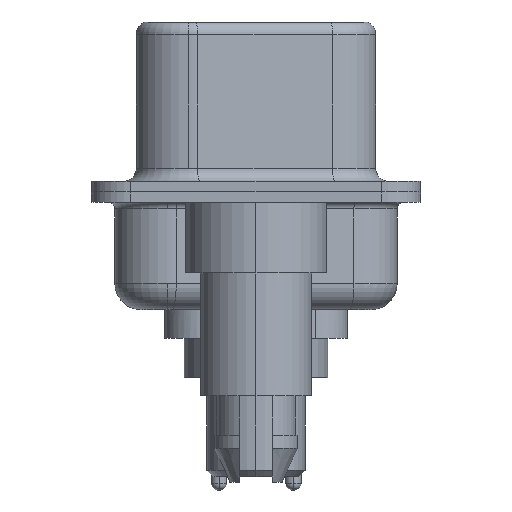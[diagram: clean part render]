
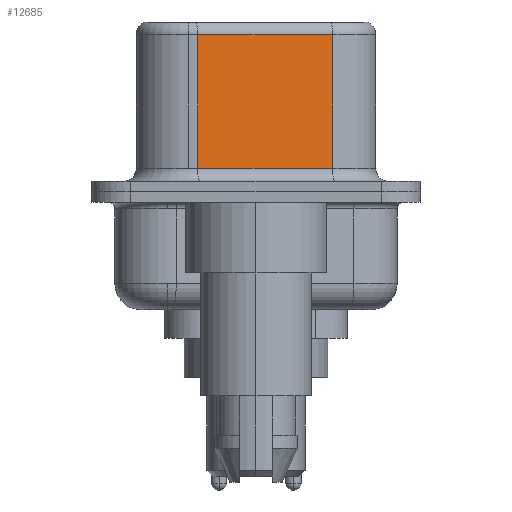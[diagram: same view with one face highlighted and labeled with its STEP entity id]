
A CAD part, left-side view. The second image highlights one B-rep face of the part: STEP entity #12685.
In plain terms, the highlighted planar face has unit normal (-0.985, -0.174, 0).
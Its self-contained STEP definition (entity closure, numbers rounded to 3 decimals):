
#523 = DIRECTION ( 'NONE',  ( -0.174, 0.985, 0. ) ) ;
#1346 = CARTESIAN_POINT ( 'NONE',  ( 4.565, -2.927, 0.9 ) ) ;
#1557 = VECTOR ( 'NONE', #4363, 1000. ) ;
#1841 = VERTEX_POINT ( 'NONE', #9374 ) ;
#3157 = LINE ( 'NONE', #1346, #6806 ) ;
#3187 = EDGE_LOOP ( 'NONE', ( #12131, #6915, #15835, #7093 ) ) ;
#3683 = CARTESIAN_POINT ( 'NONE',  ( 4.565, -2.927, 0.9 ) ) ;
#3918 = CARTESIAN_POINT ( 'NONE',  ( 4.565, -2.927, 6.02 ) ) ;
#4363 = DIRECTION ( 'NONE',  ( -0.174, 0.985, 0. ) ) ;
#4474 = VERTEX_POINT ( 'NONE', #3683 ) ;
#4487 = DIRECTION ( 'NONE',  ( 0.174, -0.985, 0. ) ) ;
#4909 = CARTESIAN_POINT ( 'NONE',  ( 3.655, 2.233, 0.9 ) ) ;
#5028 = EDGE_CURVE ( 'NONE', #8208, #1841, #9851, .T. ) ;
#5244 = EDGE_CURVE ( 'NONE', #8208, #4474, #16447, .T. ) ;
#6169 = LINE ( 'NONE', #18229, #14682 ) ;
#6806 = VECTOR ( 'NONE', #4487, 1000. ) ;
#6915 = ORIENTED_EDGE ( 'NONE', *, *, #5028, .T. ) ;
#6930 = EDGE_CURVE ( 'NONE', #1841, #20203, #6169, .T. ) ;
#7018 = DIRECTION ( 'NONE',  ( 0., 0., -1. ) ) ;
#7093 = ORIENTED_EDGE ( 'NONE', *, *, #18144, .T. ) ;
#8208 = VERTEX_POINT ( 'NONE', #3918 ) ;
#8333 = PLANE ( 'NONE',  #10334 ) ;
#9374 = CARTESIAN_POINT ( 'NONE',  ( 3.655, 2.233, 6.02 ) ) ;
#9851 = LINE ( 'NONE', #15745, #1557 ) ;
#9900 = DIRECTION ( 'NONE',  ( 0.985, 0.174, 0. ) ) ;
#10108 = DIRECTION ( 'NONE',  ( 0., 0., -1. ) ) ;
#10334 = AXIS2_PLACEMENT_3D ( 'NONE', #19604, #9900, #523 ) ;
#11743 = FACE_OUTER_BOUND ( 'NONE', #3187, .T. ) ;
#12131 = ORIENTED_EDGE ( 'NONE', *, *, #5244, .F. ) ;
#12685 = ADVANCED_FACE ( 'NONE', ( #11743 ), #8333, .F. ) ;
#14682 = VECTOR ( 'NONE', #10108, 1000. ) ;
#15432 = VECTOR ( 'NONE', #7018, 1000. ) ;
#15456 = CARTESIAN_POINT ( 'NONE',  ( 4.565, -2.927, 6.52 ) ) ;
#15745 = CARTESIAN_POINT ( 'NONE',  ( 4.565, -2.927, 6.02 ) ) ;
#15835 = ORIENTED_EDGE ( 'NONE', *, *, #6930, .T. ) ;
#16447 = LINE ( 'NONE', #15456, #15432 ) ;
#18144 = EDGE_CURVE ( 'NONE', #20203, #4474, #3157, .T. ) ;
#18229 = CARTESIAN_POINT ( 'NONE',  ( 3.655, 2.233, 6.52 ) ) ;
#19604 = CARTESIAN_POINT ( 'NONE',  ( 4.565, -2.927, 6.52 ) ) ;
#20203 = VERTEX_POINT ( 'NONE', #4909 ) ;
